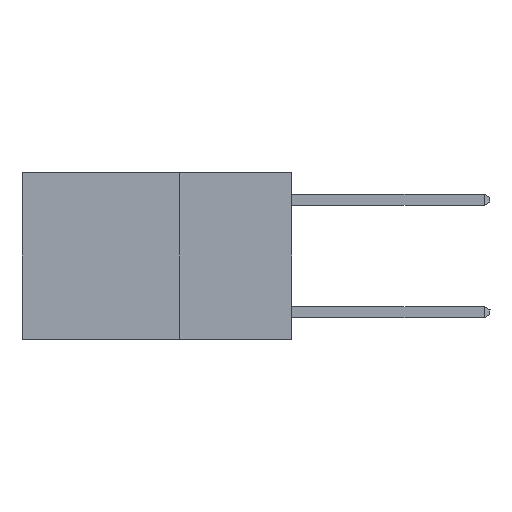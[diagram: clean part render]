
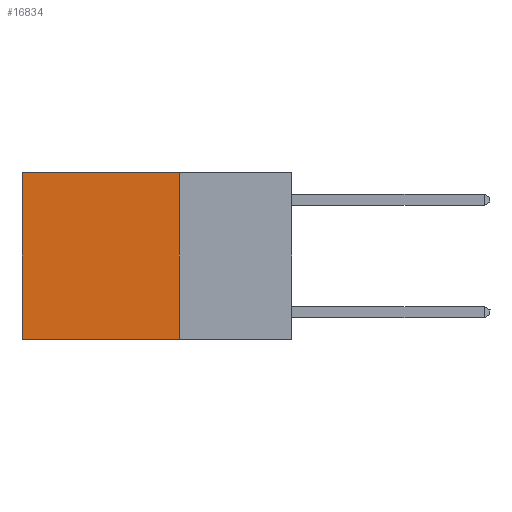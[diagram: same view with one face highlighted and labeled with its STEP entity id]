
A CAD part, left-side view. The second image highlights one B-rep face of the part: STEP entity #16834.
In plain terms, the highlighted planar face has unit normal (-1, 0, 0).
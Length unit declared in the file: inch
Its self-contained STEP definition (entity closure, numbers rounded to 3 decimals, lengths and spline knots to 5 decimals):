
#326 = EDGE_CURVE ( 'NONE', #13894, #13843, #16150, .T. ) ;
#360 = DIRECTION ( 'NONE',  ( 0., 0., -1. ) ) ;
#1034 = ORIENTED_EDGE ( 'NONE', *, *, #8457, .F. ) ;
#1236 = CARTESIAN_POINT ( 'NONE',  ( 0.2625, 0.6, 0. ) ) ;
#1284 = DIRECTION ( 'NONE',  ( 0., 1., 0. ) ) ;
#2059 = VECTOR ( 'NONE', #14593, 39.37008 ) ;
#2139 = CARTESIAN_POINT ( 'NONE',  ( 0.2625, 0.25, -0.37 ) ) ;
#2593 = EDGE_LOOP ( 'NONE', ( #15070, #5913, #1034, #10014 ) ) ;
#3411 = PLANE ( 'NONE',  #6319 ) ;
#3669 = DIRECTION ( 'NONE',  ( 0., 1., 0. ) ) ;
#4795 = VERTEX_POINT ( 'NONE', #15708 ) ;
#4951 = CARTESIAN_POINT ( 'NONE',  ( 0.2625, 0.25, 0. ) ) ;
#5551 = LINE ( 'NONE', #2139, #13546 ) ;
#5913 = ORIENTED_EDGE ( 'NONE', *, *, #11813, .F. ) ;
#6319 = AXIS2_PLACEMENT_3D ( 'NONE', #4951, #9893, #360 ) ;
#7223 = LINE ( 'NONE', #16955, #18757 ) ;
#8457 = EDGE_CURVE ( 'NONE', #13894, #4795, #18810, .T. ) ;
#8893 = CARTESIAN_POINT ( 'NONE',  ( 0.2625, 0.6, -0.37 ) ) ;
#9202 = DIRECTION ( 'NONE',  ( 0., 0., -1. ) ) ;
#9865 = EDGE_CURVE ( 'NONE', #13843, #12846, #7223, .T. ) ;
#9893 = DIRECTION ( 'NONE',  ( 1., 0., 0. ) ) ;
#10014 = ORIENTED_EDGE ( 'NONE', *, *, #326, .T. ) ;
#11563 = CARTESIAN_POINT ( 'NONE',  ( 0.2625, 0.25, 0. ) ) ;
#11813 = EDGE_CURVE ( 'NONE', #4795, #12846, #5551, .T. ) ;
#12025 = VECTOR ( 'NONE', #1284, 39.37008 ) ;
#12846 = VERTEX_POINT ( 'NONE', #8893 ) ;
#13546 = VECTOR ( 'NONE', #3669, 39.37008 ) ;
#13843 = VERTEX_POINT ( 'NONE', #1236 ) ;
#13894 = VERTEX_POINT ( 'NONE', #20148 ) ;
#14192 = FACE_OUTER_BOUND ( 'NONE', #2593, .T. ) ;
#14593 = DIRECTION ( 'NONE',  ( 0., 0., -1. ) ) ;
#15070 = ORIENTED_EDGE ( 'NONE', *, *, #9865, .T. ) ;
#15708 = CARTESIAN_POINT ( 'NONE',  ( 0.2625, 0.25, -0.37 ) ) ;
#16150 = LINE ( 'NONE', #19056, #12025 ) ;
#16834 = ADVANCED_FACE ( 'NONE', ( #14192 ), #3411, .F. ) ;
#16955 = CARTESIAN_POINT ( 'NONE',  ( 0.2625, 0.6, 0. ) ) ;
#18757 = VECTOR ( 'NONE', #9202, 39.37008 ) ;
#18810 = LINE ( 'NONE', #11563, #2059 ) ;
#19056 = CARTESIAN_POINT ( 'NONE',  ( 0.2625, 0.25, 0. ) ) ;
#20148 = CARTESIAN_POINT ( 'NONE',  ( 0.2625, 0.25, 0. ) ) ;
